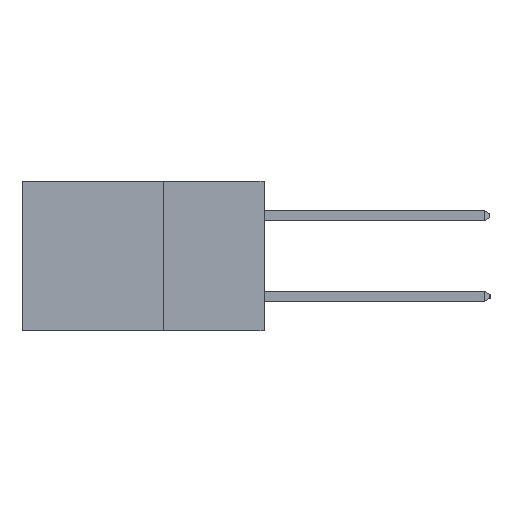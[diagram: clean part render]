
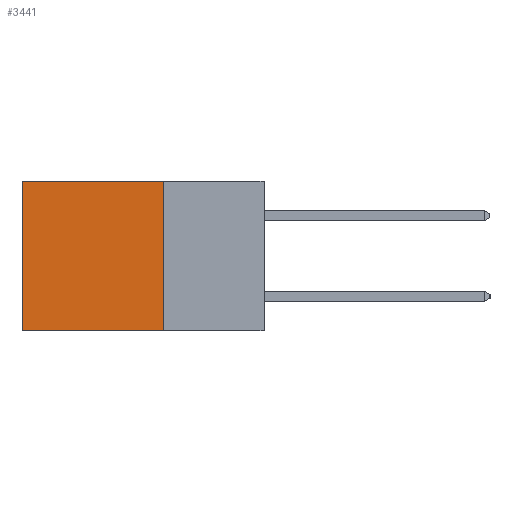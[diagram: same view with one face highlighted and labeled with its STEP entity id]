
A CAD part, left-side view. The second image highlights one B-rep face of the part: STEP entity #3441.
In plain terms, the highlighted planar face has unit normal (-1, 0, 0).
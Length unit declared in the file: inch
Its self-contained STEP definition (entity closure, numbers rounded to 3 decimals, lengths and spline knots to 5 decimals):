
#62 = EDGE_LOOP ( 'NONE', ( #9023, #9094, #9098, #9158 ) ) ;
#267 = LINE ( 'NONE', #10416, #6090 ) ;
#467 = VERTEX_POINT ( 'NONE', #5514 ) ;
#1412 = DIRECTION ( 'NONE',  ( 0., 0., -1. ) ) ;
#1754 = CARTESIAN_POINT ( 'NONE',  ( 0.2615, 0.25, -0.37 ) ) ;
#1766 = LINE ( 'NONE', #8941, #12139 ) ;
#2871 = PLANE ( 'NONE',  #12341 ) ;
#3441 = ADVANCED_FACE ( 'NONE', ( #4861 ), #2871, .F. ) ;
#3913 = VECTOR ( 'NONE', #1412, 39.37008 ) ;
#3916 = DIRECTION ( 'NONE',  ( 0., 0., -1. ) ) ;
#4186 = EDGE_CURVE ( 'NONE', #9814, #467, #1766, .T. ) ;
#4709 = DIRECTION ( 'NONE',  ( 0., 1., 0. ) ) ;
#4861 = FACE_OUTER_BOUND ( 'NONE', #62, .T. ) ;
#5514 = CARTESIAN_POINT ( 'NONE',  ( 0.2615, 0.6, -0.37 ) ) ;
#5669 = VECTOR ( 'NONE', #12316, 39.37008 ) ;
#5793 = DIRECTION ( 'NONE',  ( 1., 0., 0. ) ) ;
#6090 = VECTOR ( 'NONE', #4709, 39.37008 ) ;
#6437 = LINE ( 'NONE', #6438, #3913 ) ;
#6438 = CARTESIAN_POINT ( 'NONE',  ( 0.2615, 0.6, -0.37 ) ) ;
#7751 = CARTESIAN_POINT ( 'NONE',  ( 0.2615, 0.25, 0. ) ) ;
#8185 = LINE ( 'NONE', #10433, #5669 ) ;
#8559 = EDGE_CURVE ( 'NONE', #8802, #467, #6437, .T. ) ;
#8694 = CARTESIAN_POINT ( 'NONE',  ( 0.2615, 0.6, 0. ) ) ;
#8802 = VERTEX_POINT ( 'NONE', #8694 ) ;
#8941 = CARTESIAN_POINT ( 'NONE',  ( 0.2615, 0.25, -0.37 ) ) ;
#9023 = ORIENTED_EDGE ( 'NONE', *, *, #8559, .T. ) ;
#9094 = ORIENTED_EDGE ( 'NONE', *, *, #4186, .F. ) ;
#9098 = ORIENTED_EDGE ( 'NONE', *, *, #9720, .F. ) ;
#9158 = ORIENTED_EDGE ( 'NONE', *, *, #10369, .T. ) ;
#9611 = CARTESIAN_POINT ( 'NONE',  ( 0.2615, 0.25, -0.37 ) ) ;
#9720 = EDGE_CURVE ( 'NONE', #11177, #9814, #8185, .T. ) ;
#9814 = VERTEX_POINT ( 'NONE', #9611 ) ;
#10369 = EDGE_CURVE ( 'NONE', #11177, #8802, #267, .T. ) ;
#10416 = CARTESIAN_POINT ( 'NONE',  ( 0.2615, 0.25, 0. ) ) ;
#10433 = CARTESIAN_POINT ( 'NONE',  ( 0.2615, 0.25, -0.37 ) ) ;
#11177 = VERTEX_POINT ( 'NONE', #7751 ) ;
#12139 = VECTOR ( 'NONE', #12686, 39.37008 ) ;
#12316 = DIRECTION ( 'NONE',  ( 0., 0., -1. ) ) ;
#12341 = AXIS2_PLACEMENT_3D ( 'NONE', #1754, #5793, #3916 ) ;
#12686 = DIRECTION ( 'NONE',  ( 0., 1., 0. ) ) ;
